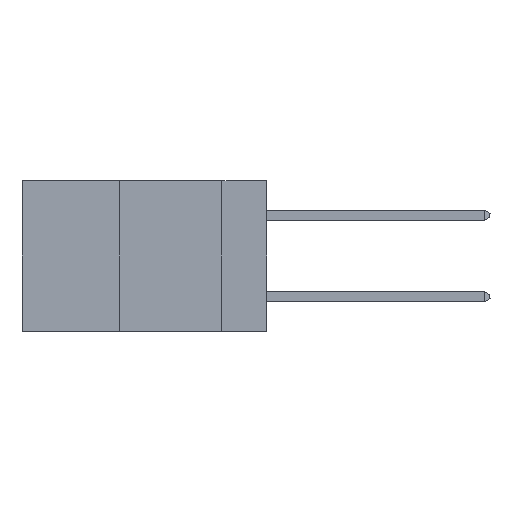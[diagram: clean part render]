
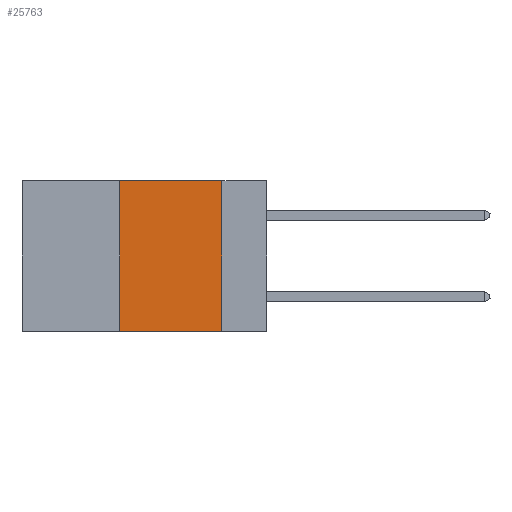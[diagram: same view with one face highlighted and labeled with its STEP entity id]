
A CAD part, left-side view. The second image highlights one B-rep face of the part: STEP entity #25763.
In plain terms, the highlighted planar face has unit normal (-1, 0, 0).
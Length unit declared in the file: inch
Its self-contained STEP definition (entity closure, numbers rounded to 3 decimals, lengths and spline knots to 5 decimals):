
#684 = AXIS2_PLACEMENT_3D ( 'NONE', #9965, #2841, #19361 ) ;
#1617 = DIRECTION ( 'NONE',  ( 0., -1., 0. ) ) ;
#2095 = VECTOR ( 'NONE', #22354, 39.37008 ) ;
#2367 = ORIENTED_EDGE ( 'NONE', *, *, #22431, .F. ) ;
#2719 = VERTEX_POINT ( 'NONE', #20138 ) ;
#2735 = PLANE ( 'NONE',  #684 ) ;
#2841 = DIRECTION ( 'NONE',  ( 1., 0., 0. ) ) ;
#2896 = EDGE_CURVE ( 'NONE', #16604, #2719, #3622, .T. ) ;
#3622 = LINE ( 'NONE', #27126, #2095 ) ;
#5573 = ORIENTED_EDGE ( 'NONE', *, *, #21456, .T. ) ;
#5772 = ORIENTED_EDGE ( 'NONE', *, *, #16511, .F. ) ;
#7701 = CARTESIAN_POINT ( 'NONE',  ( 0., 0.6, -0.37 ) ) ;
#7797 = VECTOR ( 'NONE', #28757, 39.37008 ) ;
#9965 = CARTESIAN_POINT ( 'NONE',  ( 0., 0.6, 0. ) ) ;
#10910 = CARTESIAN_POINT ( 'NONE',  ( 0., 0.36, -0.37 ) ) ;
#16146 = CARTESIAN_POINT ( 'NONE',  ( 0., 0.11, 0. ) ) ;
#16155 = VECTOR ( 'NONE', #1617, 39.37008 ) ;
#16511 = EDGE_CURVE ( 'NONE', #19388, #16604, #27815, .T. ) ;
#16604 = VERTEX_POINT ( 'NONE', #16146 ) ;
#17151 = CARTESIAN_POINT ( 'NONE',  ( 0., 0.36, 0. ) ) ;
#18209 = CARTESIAN_POINT ( 'NONE',  ( 0., 0.6, 0. ) ) ;
#18233 = DIRECTION ( 'NONE',  ( 0., 0., 1. ) ) ;
#18495 = LINE ( 'NONE', #20466, #23946 ) ;
#19361 = DIRECTION ( 'NONE',  ( 0., 0., -1. ) ) ;
#19372 = FACE_OUTER_BOUND ( 'NONE', #21045, .T. ) ;
#19388 = VERTEX_POINT ( 'NONE', #17151 ) ;
#20138 = CARTESIAN_POINT ( 'NONE',  ( 0., 0.11, -0.37 ) ) ;
#20466 = CARTESIAN_POINT ( 'NONE',  ( 0., 0.36, 0. ) ) ;
#21045 = EDGE_LOOP ( 'NONE', ( #28164, #5772, #2367, #5573 ) ) ;
#21456 = EDGE_CURVE ( 'NONE', #25334, #2719, #25734, .T. ) ;
#22354 = DIRECTION ( 'NONE',  ( 0., 0., -1. ) ) ;
#22431 = EDGE_CURVE ( 'NONE', #25334, #19388, #18495, .T. ) ;
#23946 = VECTOR ( 'NONE', #18233, 39.37008 ) ;
#25334 = VERTEX_POINT ( 'NONE', #10910 ) ;
#25734 = LINE ( 'NONE', #7701, #7797 ) ;
#25763 = ADVANCED_FACE ( 'NONE', ( #19372 ), #2735, .F. ) ;
#27126 = CARTESIAN_POINT ( 'NONE',  ( 0., 0.11, 0. ) ) ;
#27815 = LINE ( 'NONE', #18209, #16155 ) ;
#28164 = ORIENTED_EDGE ( 'NONE', *, *, #2896, .F. ) ;
#28757 = DIRECTION ( 'NONE',  ( 0., -1., 0. ) ) ;
